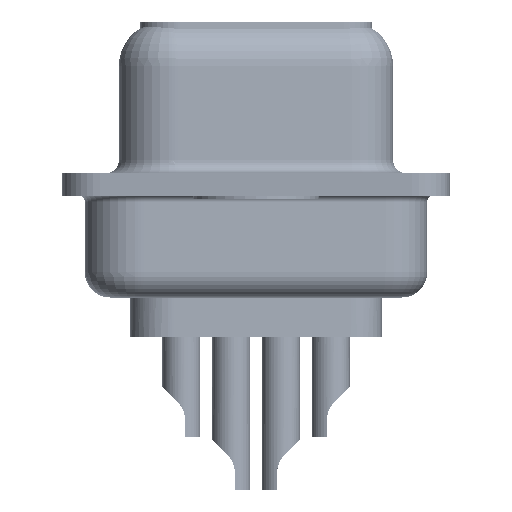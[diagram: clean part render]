
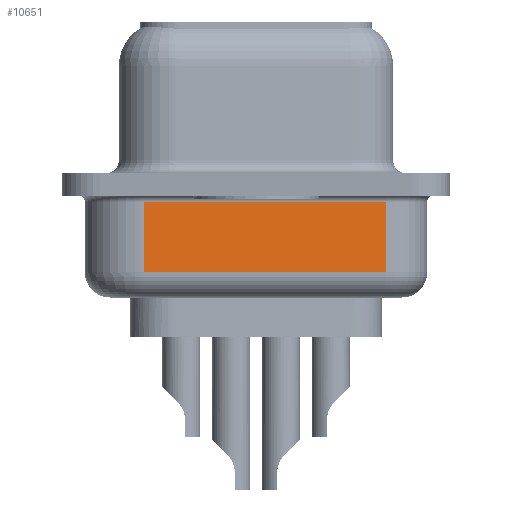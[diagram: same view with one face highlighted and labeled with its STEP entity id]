
A CAD part, left-side view. The second image highlights one B-rep face of the part: STEP entity #10651.
In plain terms, the highlighted planar face has unit normal (-0.985, -0.174, 0).
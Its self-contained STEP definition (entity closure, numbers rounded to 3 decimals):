
#798 = DIRECTION ( 'NONE',  ( 0., 0., 1. ) ) ;
#3427 = EDGE_CURVE ( 'NONE', #27275, #24974, #31514, .T. ) ;
#3755 = VECTOR ( 'NONE', #798, 1000. ) ;
#3943 = CARTESIAN_POINT ( 'NONE',  ( 3.035, 4.453, -0.7 ) ) ;
#4806 = ORIENTED_EDGE ( 'NONE', *, *, #29247, .T. ) ;
#7591 = VERTEX_POINT ( 'NONE', #49911 ) ;
#8143 = EDGE_LOOP ( 'NONE', ( #20899, #32462, #39098, #4806 ) ) ;
#9910 = CARTESIAN_POINT ( 'NONE',  ( 4.728, -5.147, -4.5 ) ) ;
#10651 = ADVANCED_FACE ( 'NONE', ( #25672 ), #14343, .F. ) ;
#12598 = CARTESIAN_POINT ( 'NONE',  ( 3.035, 4.453, -3.5 ) ) ;
#14343 = PLANE ( 'NONE',  #46921 ) ;
#14591 = CARTESIAN_POINT ( 'NONE',  ( 3.035, 4.453, -4.5 ) ) ;
#18984 = CARTESIAN_POINT ( 'NONE',  ( 4.728, -5.147, -0.7 ) ) ;
#20899 = ORIENTED_EDGE ( 'NONE', *, *, #3427, .F. ) ;
#21178 = EDGE_CURVE ( 'NONE', #27275, #7591, #42787, .T. ) ;
#21760 = LINE ( 'NONE', #9910, #45900 ) ;
#22980 = VERTEX_POINT ( 'NONE', #18984 ) ;
#24974 = VERTEX_POINT ( 'NONE', #3943 ) ;
#25657 = DIRECTION ( 'NONE',  ( -0.174, 0.985, 0. ) ) ;
#25672 = FACE_OUTER_BOUND ( 'NONE', #8143, .T. ) ;
#27275 = VERTEX_POINT ( 'NONE', #12598 ) ;
#29247 = EDGE_CURVE ( 'NONE', #22980, #24974, #45263, .T. ) ;
#29582 = DIRECTION ( 'NONE',  ( -0.174, 0.985, 0. ) ) ;
#30610 = VECTOR ( 'NONE', #40985, 1000. ) ;
#31514 = LINE ( 'NONE', #47444, #3755 ) ;
#32462 = ORIENTED_EDGE ( 'NONE', *, *, #21178, .T. ) ;
#33276 = CARTESIAN_POINT ( 'NONE',  ( 3.035, 4.453, -3.5 ) ) ;
#35826 = EDGE_CURVE ( 'NONE', #7591, #22980, #21760, .T. ) ;
#37800 = DIRECTION ( 'NONE',  ( 0.985, 0.174, 0. ) ) ;
#37990 = DIRECTION ( 'NONE',  ( 0., 0., 1. ) ) ;
#38539 = CARTESIAN_POINT ( 'NONE',  ( 3.035, 4.453, -0.7 ) ) ;
#39098 = ORIENTED_EDGE ( 'NONE', *, *, #35826, .T. ) ;
#40985 = DIRECTION ( 'NONE',  ( 0.174, -0.985, 0. ) ) ;
#42787 = LINE ( 'NONE', #33276, #30610 ) ;
#45263 = LINE ( 'NONE', #38539, #48464 ) ;
#45900 = VECTOR ( 'NONE', #37990, 1000. ) ;
#46921 = AXIS2_PLACEMENT_3D ( 'NONE', #14591, #37800, #29582 ) ;
#47444 = CARTESIAN_POINT ( 'NONE',  ( 3.035, 4.453, -4.5 ) ) ;
#48464 = VECTOR ( 'NONE', #25657, 1000. ) ;
#49911 = CARTESIAN_POINT ( 'NONE',  ( 4.728, -5.147, -3.5 ) ) ;
